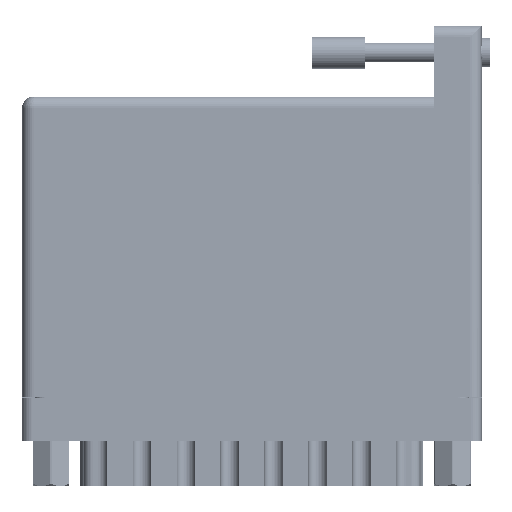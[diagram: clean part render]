
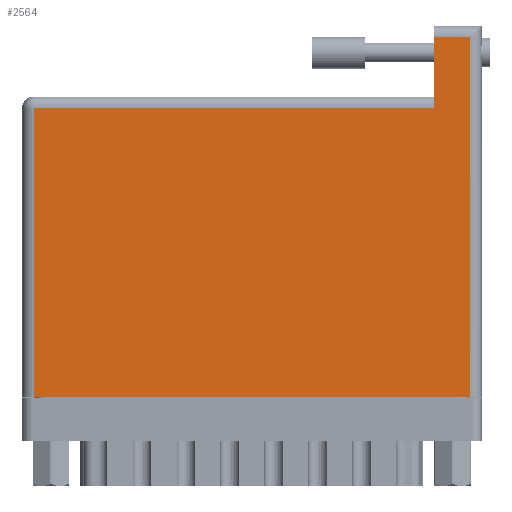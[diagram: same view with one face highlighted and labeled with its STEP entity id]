
A CAD part, front view. The second image highlights one B-rep face of the part: STEP entity #2564.
In plain terms, the highlighted face is planar.
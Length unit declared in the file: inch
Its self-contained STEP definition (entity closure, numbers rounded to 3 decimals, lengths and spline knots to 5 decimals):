
#1680 = EDGE_LOOP ( 'NONE', ( #50998, #21396, #11385, #81230, #7912, #49543 ) ) ;
#2564 = ADVANCED_FACE ( 'NONE', ( #31973 ), #49064, .F. ) ;
#5502 = DIRECTION ( 'NONE',  ( 0., -1., 0. ) ) ;
#7912 = ORIENTED_EDGE ( 'NONE', *, *, #33391, .T. ) ;
#8428 = CARTESIAN_POINT ( 'NONE',  ( 2.648, 0., 0. ) ) ;
#9480 = DIRECTION ( 'NONE',  ( 0., 0., -1. ) ) ;
#9794 = CARTESIAN_POINT ( 'NONE',  ( 2.648, 2.125, 0. ) ) ;
#10061 = VERTEX_POINT ( 'NONE', #27250 ) ;
#10354 = AXIS2_PLACEMENT_3D ( 'NONE', #82683, #9480, #69044 ) ;
#11177 = EDGE_CURVE ( 'NONE', #81263, #36946, #56191, .T. ) ;
#11311 = VERTEX_POINT ( 'NONE', #18527 ) ;
#11385 = ORIENTED_EDGE ( 'NONE', *, *, #82243, .T. ) ;
#11499 = VECTOR ( 'NONE', #5502, 39.37008 ) ;
#12516 = LINE ( 'NONE', #44832, #11499 ) ;
#12692 = CARTESIAN_POINT ( 'NONE',  ( 0., 2.125, 0. ) ) ;
#17983 = VECTOR ( 'NONE', #69736, 39.37008 ) ;
#18527 = CARTESIAN_POINT ( 'NONE',  ( 0.07, 1.705, 0. ) ) ;
#21396 = ORIENTED_EDGE ( 'NONE', *, *, #51116, .T. ) ;
#21974 = CARTESIAN_POINT ( 'NONE',  ( 0., 1.705, 0. ) ) ;
#23152 = CARTESIAN_POINT ( 'NONE',  ( 0.07, 0., 0. ) ) ;
#23784 = CARTESIAN_POINT ( 'NONE',  ( 2.648, 2.195, 0. ) ) ;
#25666 = DIRECTION ( 'NONE',  ( -1., 0., 0. ) ) ;
#25767 = CARTESIAN_POINT ( 'NONE',  ( 2.438, 2.125, 0. ) ) ;
#27250 = CARTESIAN_POINT ( 'NONE',  ( 0.07, 0., 0. ) ) ;
#28984 = DIRECTION ( 'NONE',  ( 0., -1., 0. ) ) ;
#31973 = FACE_OUTER_BOUND ( 'NONE', #1680, .T. ) ;
#33391 = EDGE_CURVE ( 'NONE', #36946, #36451, #43291, .T. ) ;
#36451 = VERTEX_POINT ( 'NONE', #25767 ) ;
#36946 = VERTEX_POINT ( 'NONE', #9794 ) ;
#42889 = DIRECTION ( 'NONE',  ( 1., 0., 0. ) ) ;
#43291 = LINE ( 'NONE', #12692, #52546 ) ;
#44548 = EDGE_CURVE ( 'NONE', #73722, #11311, #64679, .T. ) ;
#44832 = CARTESIAN_POINT ( 'NONE',  ( 2.438, 2.195, 0. ) ) ;
#44914 = VECTOR ( 'NONE', #42889, 39.37008 ) ;
#47079 = EDGE_CURVE ( 'NONE', #36451, #73722, #12516, .T. ) ;
#49064 = PLANE ( 'NONE',  #10354 ) ;
#49543 = ORIENTED_EDGE ( 'NONE', *, *, #47079, .T. ) ;
#50028 = LINE ( 'NONE', #23152, #80033 ) ;
#50998 = ORIENTED_EDGE ( 'NONE', *, *, #44548, .T. ) ;
#51116 = EDGE_CURVE ( 'NONE', #11311, #10061, #50028, .T. ) ;
#52546 = VECTOR ( 'NONE', #25666, 39.37008 ) ;
#56191 = LINE ( 'NONE', #23784, #17983 ) ;
#62016 = CARTESIAN_POINT ( 'NONE',  ( 0., 0., 0. ) ) ;
#64679 = LINE ( 'NONE', #21974, #80205 ) ;
#69044 = DIRECTION ( 'NONE',  ( -1., 0., 0. ) ) ;
#69736 = DIRECTION ( 'NONE',  ( 0., 1., 0. ) ) ;
#69824 = CARTESIAN_POINT ( 'NONE',  ( 2.438, 1.705, 0. ) ) ;
#70829 = LINE ( 'NONE', #62016, #44914 ) ;
#73722 = VERTEX_POINT ( 'NONE', #69824 ) ;
#80033 = VECTOR ( 'NONE', #28984, 39.37008 ) ;
#80205 = VECTOR ( 'NONE', #81890, 39.37008 ) ;
#81230 = ORIENTED_EDGE ( 'NONE', *, *, #11177, .T. ) ;
#81263 = VERTEX_POINT ( 'NONE', #8428 ) ;
#81890 = DIRECTION ( 'NONE',  ( -1., 0., 0. ) ) ;
#82243 = EDGE_CURVE ( 'NONE', #10061, #81263, #70829, .T. ) ;
#82683 = CARTESIAN_POINT ( 'NONE',  ( 0., 1.775, 0. ) ) ;
